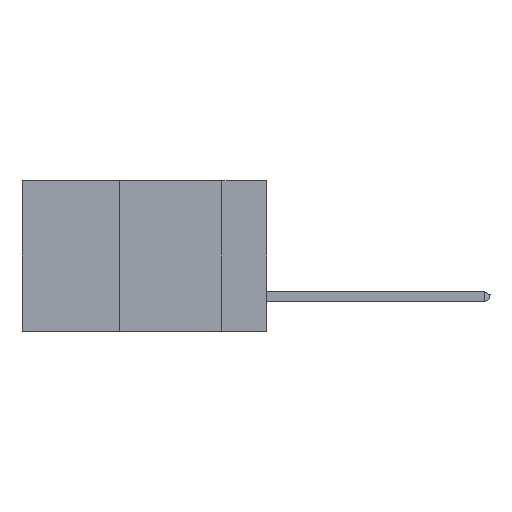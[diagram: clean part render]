
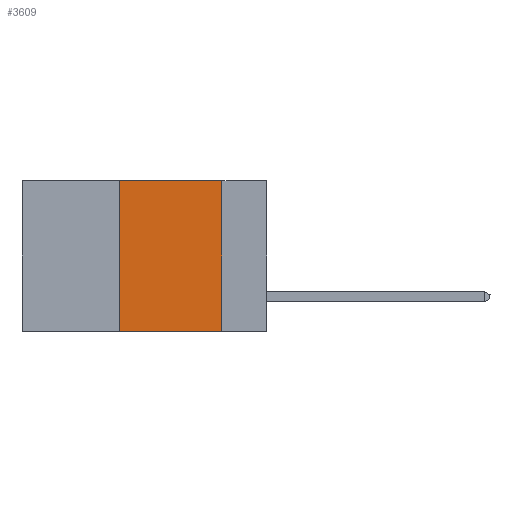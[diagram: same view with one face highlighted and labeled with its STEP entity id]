
A CAD part, left-side view. The second image highlights one B-rep face of the part: STEP entity #3609.
In plain terms, the highlighted planar face has unit normal (-1, 0, 0).
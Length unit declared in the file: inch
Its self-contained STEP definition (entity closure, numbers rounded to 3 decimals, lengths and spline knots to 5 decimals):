
#843 = VERTEX_POINT ( 'NONE', #5738 ) ;
#1843 = DIRECTION ( 'NONE',  ( 0., 0., -1. ) ) ;
#1963 = LINE ( 'NONE', #30323, #5294 ) ;
#2963 = FACE_OUTER_BOUND ( 'NONE', #14157, .T. ) ;
#3421 = VECTOR ( 'NONE', #1843, 39.37008 ) ;
#3609 = ADVANCED_FACE ( 'NONE', ( #2963 ), #29578, .F. ) ;
#4851 = CARTESIAN_POINT ( 'NONE',  ( 0., 0.6, 0. ) ) ;
#5294 = VECTOR ( 'NONE', #8725, 39.37008 ) ;
#5738 = CARTESIAN_POINT ( 'NONE',  ( 0., 0.36, -0.37 ) ) ;
#6749 = ORIENTED_EDGE ( 'NONE', *, *, #29447, .F. ) ;
#8650 = ORIENTED_EDGE ( 'NONE', *, *, #18215, .T. ) ;
#8725 = DIRECTION ( 'NONE',  ( 0., -1., 0. ) ) ;
#8912 = VECTOR ( 'NONE', #15644, 39.37008 ) ;
#10039 = ORIENTED_EDGE ( 'NONE', *, *, #29525, .F. ) ;
#11003 = LINE ( 'NONE', #30852, #3421 ) ;
#12428 = ORIENTED_EDGE ( 'NONE', *, *, #22123, .F. ) ;
#12589 = AXIS2_PLACEMENT_3D ( 'NONE', #26397, #21102, #26742 ) ;
#12928 = LINE ( 'NONE', #31645, #15030 ) ;
#14157 = EDGE_LOOP ( 'NONE', ( #6749, #10039, #12428, #8650 ) ) ;
#15030 = VECTOR ( 'NONE', #18822, 39.37008 ) ;
#15644 = DIRECTION ( 'NONE',  ( 0., -1., 0. ) ) ;
#16059 = CARTESIAN_POINT ( 'NONE',  ( 0., 0.11, 0. ) ) ;
#18215 = EDGE_CURVE ( 'NONE', #843, #33466, #1963, .T. ) ;
#18822 = DIRECTION ( 'NONE',  ( 0., 0., 1. ) ) ;
#21102 = DIRECTION ( 'NONE',  ( 1., 0., 0. ) ) ;
#22123 = EDGE_CURVE ( 'NONE', #843, #24962, #12928, .T. ) ;
#23293 = CARTESIAN_POINT ( 'NONE',  ( 0., 0.36, 0. ) ) ;
#24962 = VERTEX_POINT ( 'NONE', #23293 ) ;
#26397 = CARTESIAN_POINT ( 'NONE',  ( 0., 0.6, 0. ) ) ;
#26742 = DIRECTION ( 'NONE',  ( 0., 0., -1. ) ) ;
#29447 = EDGE_CURVE ( 'NONE', #30845, #33466, #11003, .T. ) ;
#29525 = EDGE_CURVE ( 'NONE', #24962, #30845, #30780, .T. ) ;
#29578 = PLANE ( 'NONE',  #12589 ) ;
#30323 = CARTESIAN_POINT ( 'NONE',  ( 0., 0.6, -0.37 ) ) ;
#30780 = LINE ( 'NONE', #4851, #8912 ) ;
#30845 = VERTEX_POINT ( 'NONE', #16059 ) ;
#30852 = CARTESIAN_POINT ( 'NONE',  ( 0., 0.11, 0. ) ) ;
#31132 = CARTESIAN_POINT ( 'NONE',  ( 0., 0.11, -0.37 ) ) ;
#31645 = CARTESIAN_POINT ( 'NONE',  ( 0., 0.36, 0. ) ) ;
#33466 = VERTEX_POINT ( 'NONE', #31132 ) ;
